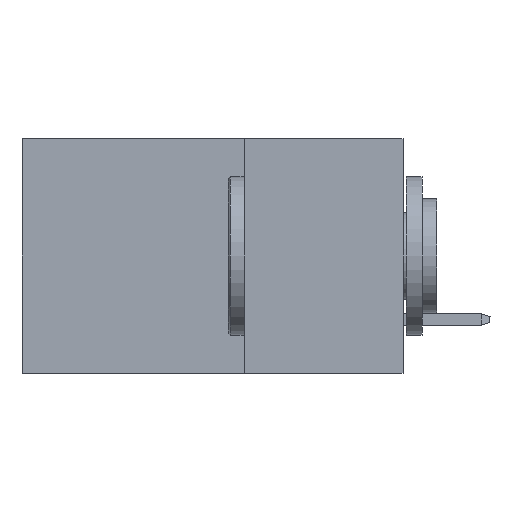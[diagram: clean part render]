
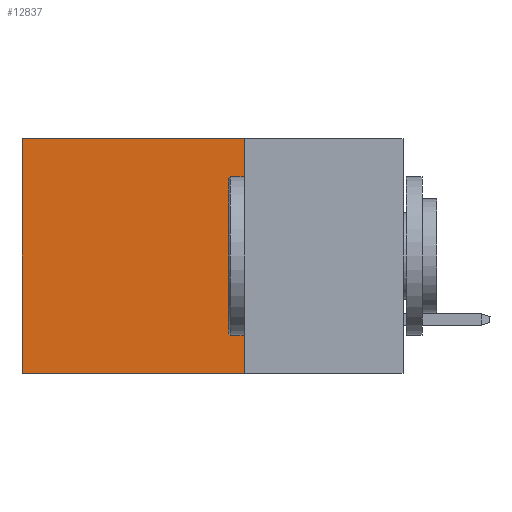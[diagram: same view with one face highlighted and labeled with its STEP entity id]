
A CAD part, left-side view. The second image highlights one B-rep face of the part: STEP entity #12837.
In plain terms, the highlighted planar face has unit normal (-1, 0, 0).
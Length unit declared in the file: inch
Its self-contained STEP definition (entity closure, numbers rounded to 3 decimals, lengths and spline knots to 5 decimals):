
#123 = VERTEX_POINT ( 'NONE', #17200 ) ;
#385 = LINE ( 'NONE', #17860, #6826 ) ;
#596 = CARTESIAN_POINT ( 'NONE',  ( 0.2875, 0.25, 0. ) ) ;
#980 = ORIENTED_EDGE ( 'NONE', *, *, #7727, .T. ) ;
#1098 = EDGE_LOOP ( 'NONE', ( #980, #12652, #16208, #4377 ) ) ;
#1825 = CARTESIAN_POINT ( 'NONE',  ( 0.2875, 0.25, -0.37 ) ) ;
#2578 = VECTOR ( 'NONE', #2868, 39.37008 ) ;
#2786 = DIRECTION ( 'NONE',  ( 0., 0., -1. ) ) ;
#2868 = DIRECTION ( 'NONE',  ( 0., 0., -1. ) ) ;
#3965 = LINE ( 'NONE', #1825, #15638 ) ;
#4377 = ORIENTED_EDGE ( 'NONE', *, *, #13432, .T. ) ;
#6270 = PLANE ( 'NONE',  #7404 ) ;
#6307 = LINE ( 'NONE', #6585, #6540 ) ;
#6451 = DIRECTION ( 'NONE',  ( 0., 1., 0. ) ) ;
#6540 = VECTOR ( 'NONE', #6451, 39.37008 ) ;
#6585 = CARTESIAN_POINT ( 'NONE',  ( 0.2875, 0.25, 0. ) ) ;
#6826 = VECTOR ( 'NONE', #2786, 39.37008 ) ;
#7404 = AXIS2_PLACEMENT_3D ( 'NONE', #19223, #8431, #17106 ) ;
#7727 = EDGE_CURVE ( 'NONE', #22581, #123, #385, .T. ) ;
#8431 = DIRECTION ( 'NONE',  ( 1., 0., 0. ) ) ;
#10513 = CARTESIAN_POINT ( 'NONE',  ( 0.2875, 0.25, 0. ) ) ;
#11828 = VERTEX_POINT ( 'NONE', #10513 ) ;
#12652 = ORIENTED_EDGE ( 'NONE', *, *, #18745, .F. ) ;
#12837 = ADVANCED_FACE ( 'NONE', ( #16969 ), #6270, .F. ) ;
#13432 = EDGE_CURVE ( 'NONE', #11828, #22581, #6307, .T. ) ;
#15638 = VECTOR ( 'NONE', #25803, 39.37008 ) ;
#16208 = ORIENTED_EDGE ( 'NONE', *, *, #23309, .F. ) ;
#16969 = FACE_OUTER_BOUND ( 'NONE', #1098, .T. ) ;
#17106 = DIRECTION ( 'NONE',  ( 0., 0., -1. ) ) ;
#17200 = CARTESIAN_POINT ( 'NONE',  ( 0.2875, 0.6, -0.37 ) ) ;
#17860 = CARTESIAN_POINT ( 'NONE',  ( 0.2875, 0.6, 0. ) ) ;
#18745 = EDGE_CURVE ( 'NONE', #25854, #123, #3965, .T. ) ;
#19223 = CARTESIAN_POINT ( 'NONE',  ( 0.2875, 0.25, 0. ) ) ;
#22298 = LINE ( 'NONE', #596, #2578 ) ;
#22581 = VERTEX_POINT ( 'NONE', #27476 ) ;
#23309 = EDGE_CURVE ( 'NONE', #11828, #25854, #22298, .T. ) ;
#23425 = CARTESIAN_POINT ( 'NONE',  ( 0.2875, 0.25, -0.37 ) ) ;
#25803 = DIRECTION ( 'NONE',  ( 0., 1., 0. ) ) ;
#25854 = VERTEX_POINT ( 'NONE', #23425 ) ;
#27476 = CARTESIAN_POINT ( 'NONE',  ( 0.2875, 0.6, 0. ) ) ;
